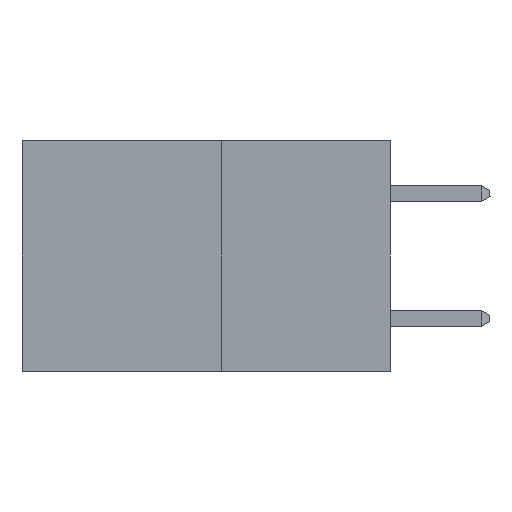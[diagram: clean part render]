
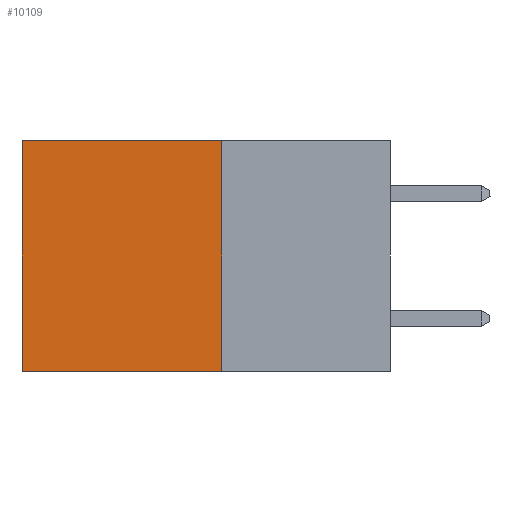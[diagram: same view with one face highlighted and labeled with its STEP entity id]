
A CAD part, left-side view. The second image highlights one B-rep face of the part: STEP entity #10109.
In plain terms, the highlighted planar face has unit normal (-1, 0, 0).
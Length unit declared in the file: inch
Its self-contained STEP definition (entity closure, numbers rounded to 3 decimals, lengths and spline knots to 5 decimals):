
#312 = VECTOR ( 'NONE', #9364, 39.37008 ) ;
#1083 = DIRECTION ( 'NONE',  ( 0., 1., 0. ) ) ;
#1661 = ORIENTED_EDGE ( 'NONE', *, *, #11227, .T. ) ;
#1724 = PLANE ( 'NONE',  #17078 ) ;
#3153 = VERTEX_POINT ( 'NONE', #4737 ) ;
#3275 = DIRECTION ( 'NONE',  ( 0., 0., -1. ) ) ;
#4066 = LINE ( 'NONE', #16184, #11591 ) ;
#4336 = CARTESIAN_POINT ( 'NONE',  ( 0.277, 0.59, -0.37 ) ) ;
#4737 = CARTESIAN_POINT ( 'NONE',  ( 0.277, 0.59, 0. ) ) ;
#5091 = CARTESIAN_POINT ( 'NONE',  ( 0.277, 0.27, 0. ) ) ;
#5529 = EDGE_CURVE ( 'NONE', #11678, #8381, #4066, .T. ) ;
#8381 = VERTEX_POINT ( 'NONE', #17363 ) ;
#8464 = VECTOR ( 'NONE', #1083, 39.37008 ) ;
#9280 = ORIENTED_EDGE ( 'NONE', *, *, #17227, .F. ) ;
#9364 = DIRECTION ( 'NONE',  ( 0., 1., 0. ) ) ;
#10109 = ADVANCED_FACE ( 'NONE', ( #17088 ), #1724, .F. ) ;
#10617 = EDGE_CURVE ( 'NONE', #3153, #15648, #11771, .T. ) ;
#10818 = DIRECTION ( 'NONE',  ( 0., 0., -1. ) ) ;
#11227 = EDGE_CURVE ( 'NONE', #11678, #3153, #17269, .T. ) ;
#11591 = VECTOR ( 'NONE', #10818, 39.37008 ) ;
#11671 = CARTESIAN_POINT ( 'NONE',  ( 0.277, 0.27, 0. ) ) ;
#11678 = VERTEX_POINT ( 'NONE', #5091 ) ;
#11771 = LINE ( 'NONE', #4336, #15221 ) ;
#12281 = DIRECTION ( 'NONE',  ( 1., 0., 0. ) ) ;
#13174 = ORIENTED_EDGE ( 'NONE', *, *, #5529, .F. ) ;
#13898 = EDGE_LOOP ( 'NONE', ( #16206, #9280, #13174, #1661 ) ) ;
#15221 = VECTOR ( 'NONE', #16270, 39.37008 ) ;
#15288 = CARTESIAN_POINT ( 'NONE',  ( 0.277, 0.59, -0.37 ) ) ;
#15648 = VERTEX_POINT ( 'NONE', #15288 ) ;
#16184 = CARTESIAN_POINT ( 'NONE',  ( 0.277, 0.27, -0.37 ) ) ;
#16206 = ORIENTED_EDGE ( 'NONE', *, *, #10617, .T. ) ;
#16270 = DIRECTION ( 'NONE',  ( 0., 0., -1. ) ) ;
#16299 = LINE ( 'NONE', #16733, #312 ) ;
#16733 = CARTESIAN_POINT ( 'NONE',  ( 0.277, 0.27, -0.37 ) ) ;
#17078 = AXIS2_PLACEMENT_3D ( 'NONE', #18088, #12281, #3275 ) ;
#17088 = FACE_OUTER_BOUND ( 'NONE', #13898, .T. ) ;
#17227 = EDGE_CURVE ( 'NONE', #8381, #15648, #16299, .T. ) ;
#17269 = LINE ( 'NONE', #11671, #8464 ) ;
#17363 = CARTESIAN_POINT ( 'NONE',  ( 0.277, 0.27, -0.37 ) ) ;
#18088 = CARTESIAN_POINT ( 'NONE',  ( 0.277, 0.27, -0.37 ) ) ;
